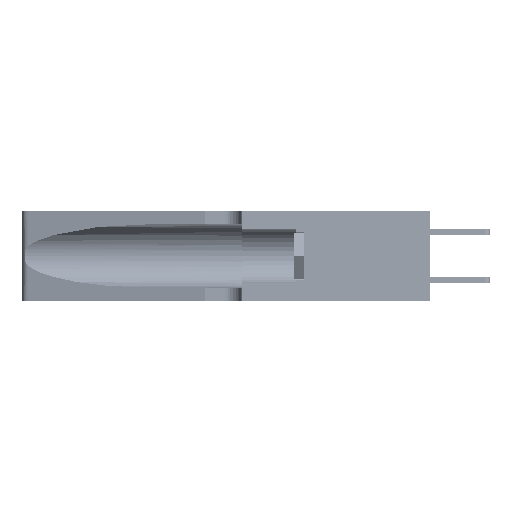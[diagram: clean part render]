
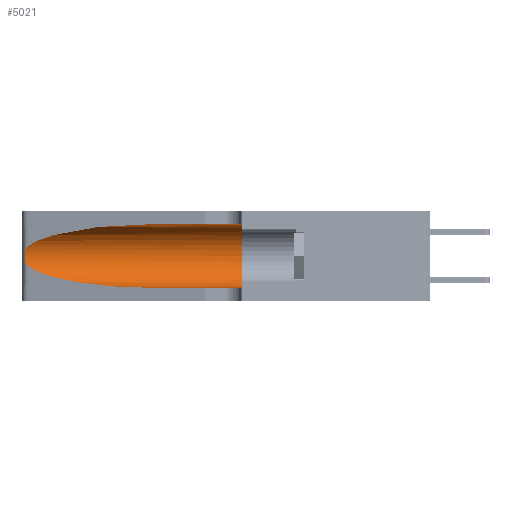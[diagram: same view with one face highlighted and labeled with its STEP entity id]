
A CAD part, left-side view. The second image highlights one B-rep face of the part: STEP entity #5021.
In plain terms, the highlighted cylindrical face has radius 3.308 mm (diameter 6.617 mm), a partial arc.
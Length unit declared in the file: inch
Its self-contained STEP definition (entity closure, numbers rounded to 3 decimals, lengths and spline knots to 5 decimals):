
#390 =( BOUNDED_CURVE ( )  B_SPLINE_CURVE ( 3, ( #33767, #20840, #1392, #6009 ),
 .UNSPECIFIED., .F., .F. ) 
 B_SPLINE_CURVE_WITH_KNOTS ( ( 4, 4 ),
 ( 1.5708, 2.84003 ),
 .UNSPECIFIED. ) 
 CURVE ( )  GEOMETRIC_REPRESENTATION_ITEM ( )  RATIONAL_B_SPLINE_CURVE ( ( 1., 0.87, 0.87, 1. ) ) 
 REPRESENTATION_ITEM ( '' )  );
#397 = CARTESIAN_POINT ( 'NONE',  ( 0.1305, 0.35, 0.05475 ) ) ;
#1392 = CARTESIAN_POINT ( 'NONE',  ( 0.2373, 1.15595, 0.28018 ) ) ;
#3498 = CARTESIAN_POINT ( 'NONE',  ( 0.25856, 1.23593, 0.16098 ) ) ;
#4560 = FACE_OUTER_BOUND ( 'NONE', #43243, .T. ) ;
#4617 = EDGE_CURVE ( 'NONE', #25609, #26659, #390, .T. ) ;
#5021 = ADVANCED_FACE ( 'NONE', ( #4560 ), #43554, .F. ) ;
#5127 = CARTESIAN_POINT ( 'NONE',  ( 0.1305, 1.61858, 0.31525 ) ) ;
#5351 = CARTESIAN_POINT ( 'NONE',  ( 0.1305, 0.35, 0.185 ) ) ;
#5844 = CARTESIAN_POINT ( 'NONE',  ( 0.1305, 1.61858, 0.185 ) ) ;
#6009 = CARTESIAN_POINT ( 'NONE',  ( 0.25487, 1.22718, 0.22369 ) ) ;
#7171 = CARTESIAN_POINT ( 'NONE',  ( 0.25789, 1.23486, 0.15765 ) ) ;
#7635 = CARTESIAN_POINT ( 'NONE',  ( 0.25639, 1.23186, 0.15144 ) ) ;
#8084 = DIRECTION ( 'NONE',  ( 0., -1., 0. ) ) ;
#9851 = LINE ( 'NONE', #19302, #19820 ) ;
#10449 = CARTESIAN_POINT ( 'NONE',  ( 0.1305, 0.35, 0.31525 ) ) ;
#10630 = CIRCLE ( 'NONE', #19796, 0.13025 ) ;
#10802 = CARTESIAN_POINT ( 'NONE',  ( 0.26075, 1.23896, 0.19203 ) ) ;
#11120 = CARTESIAN_POINT ( 'NONE',  ( 0.25487, 1.22718, 0.22369 ) ) ;
#11272 = CARTESIAN_POINT ( 'NONE',  ( 0.25555, 1.22994, 0.2215 ) ) ;
#11579 =( BOUNDED_CURVE ( )  B_SPLINE_CURVE ( 3, ( #35586, #35911, #43157, #20878 ),
 .UNSPECIFIED., .F., .F. ) 
 B_SPLINE_CURVE_WITH_KNOTS ( ( 4, 4 ),
 ( 3.44316, 4.71239 ),
 .UNSPECIFIED. ) 
 CURVE ( )  GEOMETRIC_REPRESENTATION_ITEM ( )  RATIONAL_B_SPLINE_CURVE ( ( 1., 0.87, 0.87, 1. ) ) 
 REPRESENTATION_ITEM ( '' )  );
#12221 = ORIENTED_EDGE ( 'NONE', *, *, #27593, .T. ) ;
#12884 = DIRECTION ( 'NONE',  ( 0., -1., 0. ) ) ;
#12931 = DIRECTION ( 'NONE',  ( 0., 1., 0. ) ) ;
#13557 = VERTEX_POINT ( 'NONE', #10449 ) ;
#14556 = VERTEX_POINT ( 'NONE', #397 ) ;
#14580 = CARTESIAN_POINT ( 'NONE',  ( 0.26017, 1.23833, 0.17102 ) ) ;
#15050 = CARTESIAN_POINT ( 'NONE',  ( 0.25787, 1.23484, 0.2124 ) ) ;
#19302 = CARTESIAN_POINT ( 'NONE',  ( 0.1305, 1.61858, 0.05475 ) ) ;
#19796 = AXIS2_PLACEMENT_3D ( 'NONE', #5351, #12931, #39347 ) ;
#19820 = VECTOR ( 'NONE', #8084, 39.37008 ) ;
#20069 = AXIS2_PLACEMENT_3D ( 'NONE', #5844, #36693, #32270 ) ;
#20840 = CARTESIAN_POINT ( 'NONE',  ( 0.18966, 0.96281, 0.31525 ) ) ;
#20878 = CARTESIAN_POINT ( 'NONE',  ( 0.1305, 0.72297, 0.05475 ) ) ;
#21711 = EDGE_CURVE ( 'NONE', #25609, #13557, #28923, .T. ) ;
#22463 = CARTESIAN_POINT ( 'NONE',  ( 0.25639, 1.23184, 0.21858 ) ) ;
#25609 = VERTEX_POINT ( 'NONE', #41734 ) ;
#26425 = CARTESIAN_POINT ( 'NONE',  ( 0.25555, 1.22993, 0.14849 ) ) ;
#26659 = VERTEX_POINT ( 'NONE', #43143 ) ;
#27593 = EDGE_CURVE ( 'NONE', #28472, #14556, #9851, .T. ) ;
#27602 = B_SPLINE_CURVE_WITH_KNOTS ( 'NONE', 3,
 ( #11120, #11272, #22463, #15050, #48542, #37798, #10802, #33562, #14580, #3498, #7171, #7635, #26425, #41291 ),
 .UNSPECIFIED., .F., .F.,
 ( 4, 2, 2, 2, 2, 2, 4 ),
 ( 0., 0.00027, 0.00053, 0.00107, 0.0016, 0.00187, 0.00214 ),
 .UNSPECIFIED. ) ;
#28472 = VERTEX_POINT ( 'NONE', #31237 ) ;
#28923 = LINE ( 'NONE', #5127, #37169 ) ;
#30707 = CARTESIAN_POINT ( 'NONE',  ( 0.25487, 1.22718, 0.14631 ) ) ;
#31237 = CARTESIAN_POINT ( 'NONE',  ( 0.1305, 0.72297, 0.05475 ) ) ;
#31293 = ORIENTED_EDGE ( 'NONE', *, *, #32208, .T. ) ;
#31397 = EDGE_CURVE ( 'NONE', #36447, #28472, #11579, .T. ) ;
#31750 = ORIENTED_EDGE ( 'NONE', *, *, #31397, .T. ) ;
#32208 = EDGE_CURVE ( 'NONE', #26659, #36447, #27602, .T. ) ;
#32270 = DIRECTION ( 'NONE',  ( 0., 0., -1. ) ) ;
#33562 = CARTESIAN_POINT ( 'NONE',  ( 0.26075, 1.23896, 0.178 ) ) ;
#33767 = CARTESIAN_POINT ( 'NONE',  ( 0.1305, 0.72297, 0.31525 ) ) ;
#35586 = CARTESIAN_POINT ( 'NONE',  ( 0.25487, 1.22718, 0.14631 ) ) ;
#35911 = CARTESIAN_POINT ( 'NONE',  ( 0.2373, 1.15595, 0.08982 ) ) ;
#36447 = VERTEX_POINT ( 'NONE', #30707 ) ;
#36693 = DIRECTION ( 'NONE',  ( 0., -1., 0. ) ) ;
#37169 = VECTOR ( 'NONE', #12884, 39.37008 ) ;
#37798 = CARTESIAN_POINT ( 'NONE',  ( 0.26018, 1.23835, 0.19895 ) ) ;
#39347 = DIRECTION ( 'NONE',  ( 0., 0., 1. ) ) ;
#39369 = ORIENTED_EDGE ( 'NONE', *, *, #45998, .F. ) ;
#40741 = ORIENTED_EDGE ( 'NONE', *, *, #4617, .T. ) ;
#41291 = CARTESIAN_POINT ( 'NONE',  ( 0.25487, 1.22718, 0.14631 ) ) ;
#41734 = CARTESIAN_POINT ( 'NONE',  ( 0.1305, 0.72297, 0.31525 ) ) ;
#43143 = CARTESIAN_POINT ( 'NONE',  ( 0.25487, 1.22718, 0.22369 ) ) ;
#43157 = CARTESIAN_POINT ( 'NONE',  ( 0.18966, 0.96281, 0.05475 ) ) ;
#43243 = EDGE_LOOP ( 'NONE', ( #40741, #31293, #31750, #12221, #39369, #44791 ) ) ;
#43554 = CYLINDRICAL_SURFACE ( 'NONE', #20069, 0.13025 ) ;
#44791 = ORIENTED_EDGE ( 'NONE', *, *, #21711, .F. ) ;
#45998 = EDGE_CURVE ( 'NONE', #13557, #14556, #10630, .T. ) ;
#48542 = CARTESIAN_POINT ( 'NONE',  ( 0.25854, 1.2359, 0.20912 ) ) ;
